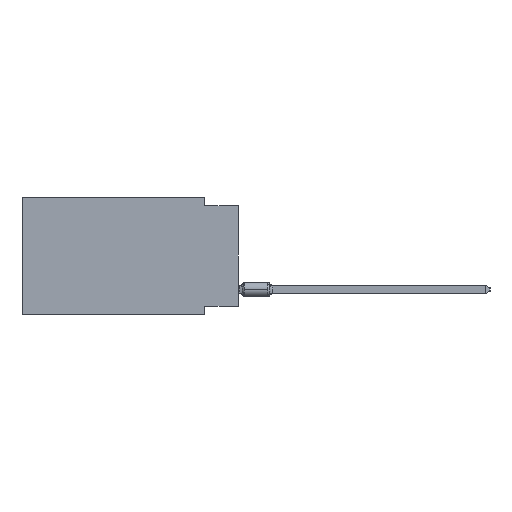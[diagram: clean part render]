
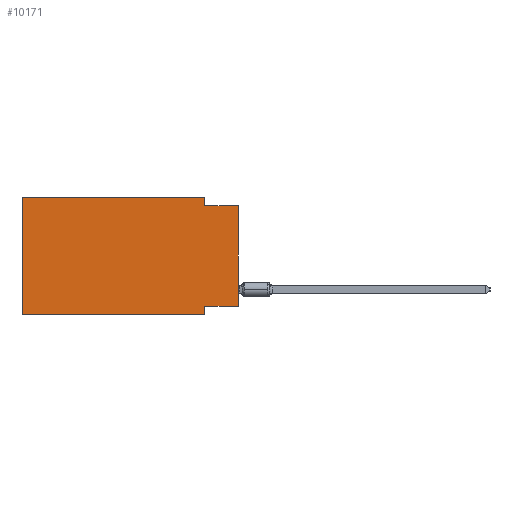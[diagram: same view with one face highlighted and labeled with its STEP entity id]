
A CAD part, left-side view. The second image highlights one B-rep face of the part: STEP entity #10171.
In plain terms, the highlighted planar face has unit normal (-1, 0, 0).
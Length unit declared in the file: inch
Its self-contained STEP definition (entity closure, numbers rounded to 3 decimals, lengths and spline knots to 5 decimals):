
#749 = VERTEX_POINT ( 'NONE', #10912 ) ;
#1488 = CARTESIAN_POINT ( 'NONE',  ( 0., 0., 0. ) ) ;
#1971 = EDGE_CURVE ( 'NONE', #7661, #8246, #28090, .T. ) ;
#2269 = EDGE_CURVE ( 'NONE', #17874, #7654, #8333, .T. ) ;
#2424 = CARTESIAN_POINT ( 'NONE',  ( 0., 0.645, 0. ) ) ;
#2901 = VECTOR ( 'NONE', #28947, 39.37008 ) ;
#4229 = VECTOR ( 'NONE', #38660, 39.37008 ) ;
#4399 = VECTOR ( 'NONE', #36933, 39.37008 ) ;
#5844 = CARTESIAN_POINT ( 'NONE',  ( 0., 0., -0.325 ) ) ;
#6027 = VECTOR ( 'NONE', #37890, 39.37008 ) ;
#7440 = ORIENTED_EDGE ( 'NONE', *, *, #14944, .T. ) ;
#7654 = VERTEX_POINT ( 'NONE', #28223 ) ;
#7661 = VERTEX_POINT ( 'NONE', #13858 ) ;
#8246 = VERTEX_POINT ( 'NONE', #34833 ) ;
#8333 = LINE ( 'NONE', #8804, #4399 ) ;
#8804 = CARTESIAN_POINT ( 'NONE',  ( 0., 0.645, 0. ) ) ;
#9536 = CARTESIAN_POINT ( 'NONE',  ( 0., 0., -0.025 ) ) ;
#9740 = CARTESIAN_POINT ( 'NONE',  ( 0., 0.1, -0.325 ) ) ;
#10117 = ORIENTED_EDGE ( 'NONE', *, *, #17714, .F. ) ;
#10171 = ADVANCED_FACE ( 'NONE', ( #42793 ), #43498, .F. ) ;
#10912 = CARTESIAN_POINT ( 'NONE',  ( 0., 0.1, -0.35 ) ) ;
#11951 = LINE ( 'NONE', #1488, #33556 ) ;
#12316 = VERTEX_POINT ( 'NONE', #9740 ) ;
#13218 = ORIENTED_EDGE ( 'NONE', *, *, #2269, .F. ) ;
#13858 = CARTESIAN_POINT ( 'NONE',  ( 0., 0.1, -0.025 ) ) ;
#14944 = EDGE_CURVE ( 'NONE', #35339, #8246, #11951, .T. ) ;
#16802 = CARTESIAN_POINT ( 'NONE',  ( 0., 0.1, 0. ) ) ;
#17628 = EDGE_CURVE ( 'NONE', #17874, #749, #18498, .T. ) ;
#17714 = EDGE_CURVE ( 'NONE', #12316, #749, #18013, .T. ) ;
#17720 = LINE ( 'NONE', #16802, #4229 ) ;
#17766 = DIRECTION ( 'NONE',  ( 0., 1., 0. ) ) ;
#17874 = VERTEX_POINT ( 'NONE', #34671 ) ;
#18013 = LINE ( 'NONE', #39421, #2901 ) ;
#18498 = LINE ( 'NONE', #24749, #37773 ) ;
#19153 = DIRECTION ( 'NONE',  ( 0., 0., 1. ) ) ;
#19425 = EDGE_LOOP ( 'NONE', ( #7440, #29254, #24557, #36022, #13218, #44892, #10117, #41850 ) ) ;
#22262 = LINE ( 'NONE', #2424, #26235 ) ;
#23728 = EDGE_CURVE ( 'NONE', #35339, #12316, #41963, .T. ) ;
#24557 = ORIENTED_EDGE ( 'NONE', *, *, #35098, .F. ) ;
#24749 = CARTESIAN_POINT ( 'NONE',  ( 0., 0.645, -0.35 ) ) ;
#24963 = CARTESIAN_POINT ( 'NONE',  ( 0., 0., -0.325 ) ) ;
#26235 = VECTOR ( 'NONE', #40167, 39.37008 ) ;
#28090 = LINE ( 'NONE', #9536, #6027 ) ;
#28223 = CARTESIAN_POINT ( 'NONE',  ( 0., 0.645, 0. ) ) ;
#28594 = DIRECTION ( 'NONE',  ( 0., 0., -1. ) ) ;
#28709 = DIRECTION ( 'NONE',  ( 0., -1., 0. ) ) ;
#28825 = DIRECTION ( 'NONE',  ( 1., 0., 0. ) ) ;
#28900 = CARTESIAN_POINT ( 'NONE',  ( 0., 0.1, 0. ) ) ;
#28947 = DIRECTION ( 'NONE',  ( 0., 0., -1. ) ) ;
#29254 = ORIENTED_EDGE ( 'NONE', *, *, #1971, .F. ) ;
#30069 = VERTEX_POINT ( 'NONE', #28900 ) ;
#31826 = EDGE_CURVE ( 'NONE', #7654, #30069, #22262, .T. ) ;
#32546 = AXIS2_PLACEMENT_3D ( 'NONE', #39317, #28825, #28594 ) ;
#33556 = VECTOR ( 'NONE', #19153, 39.37008 ) ;
#34671 = CARTESIAN_POINT ( 'NONE',  ( 0., 0.645, -0.35 ) ) ;
#34833 = CARTESIAN_POINT ( 'NONE',  ( 0., 0., -0.025 ) ) ;
#35098 = EDGE_CURVE ( 'NONE', #30069, #7661, #17720, .T. ) ;
#35339 = VERTEX_POINT ( 'NONE', #5844 ) ;
#36022 = ORIENTED_EDGE ( 'NONE', *, *, #31826, .F. ) ;
#36933 = DIRECTION ( 'NONE',  ( 0., 0., 1. ) ) ;
#37773 = VECTOR ( 'NONE', #28709, 39.37008 ) ;
#37890 = DIRECTION ( 'NONE',  ( 0., -1., 0. ) ) ;
#38104 = VECTOR ( 'NONE', #17766, 39.37008 ) ;
#38660 = DIRECTION ( 'NONE',  ( 0., 0., -1. ) ) ;
#39317 = CARTESIAN_POINT ( 'NONE',  ( 0., 0.645, 0. ) ) ;
#39421 = CARTESIAN_POINT ( 'NONE',  ( 0., 0.1, -0.35 ) ) ;
#40167 = DIRECTION ( 'NONE',  ( 0., -1., 0. ) ) ;
#41850 = ORIENTED_EDGE ( 'NONE', *, *, #23728, .F. ) ;
#41963 = LINE ( 'NONE', #24963, #38104 ) ;
#42793 = FACE_OUTER_BOUND ( 'NONE', #19425, .T. ) ;
#43498 = PLANE ( 'NONE',  #32546 ) ;
#44892 = ORIENTED_EDGE ( 'NONE', *, *, #17628, .T. ) ;
